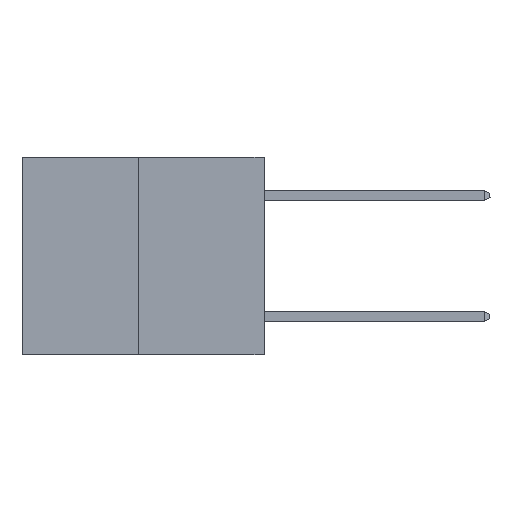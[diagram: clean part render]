
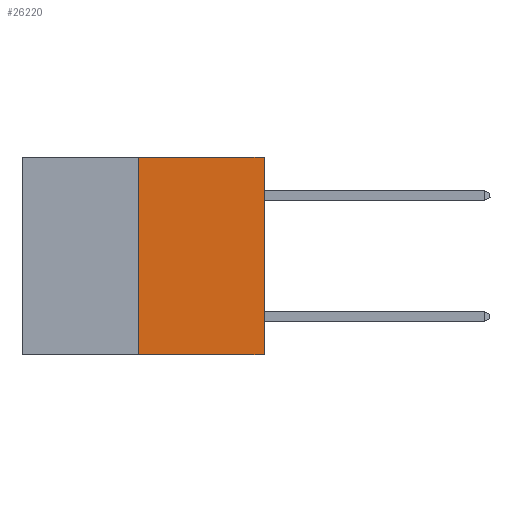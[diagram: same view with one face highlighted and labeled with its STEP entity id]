
A CAD part, left-side view. The second image highlights one B-rep face of the part: STEP entity #26220.
In plain terms, the highlighted planar face has unit normal (-1, 0, 0).
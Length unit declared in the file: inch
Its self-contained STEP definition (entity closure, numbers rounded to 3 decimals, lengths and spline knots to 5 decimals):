
#441 = LINE ( 'NONE', #14426, #9170 ) ;
#794 = DIRECTION ( 'NONE',  ( 1., 0., 0. ) ) ;
#1610 = LINE ( 'NONE', #24956, #11942 ) ;
#2062 = DIRECTION ( 'NONE',  ( 0., -1., 0. ) ) ;
#3637 = EDGE_CURVE ( 'NONE', #22764, #22365, #1610, .T. ) ;
#3825 = CARTESIAN_POINT ( 'NONE',  ( 0., 0., -0.49 ) ) ;
#4511 = ORIENTED_EDGE ( 'NONE', *, *, #6900, .F. ) ;
#5049 = ORIENTED_EDGE ( 'NONE', *, *, #18432, .T. ) ;
#6900 = EDGE_CURVE ( 'NONE', #22365, #22839, #441, .T. ) ;
#8186 = CARTESIAN_POINT ( 'NONE',  ( 0., 0., 0. ) ) ;
#9100 = VECTOR ( 'NONE', #10522, 39.37008 ) ;
#9170 = VECTOR ( 'NONE', #2062, 39.37008 ) ;
#10032 = EDGE_CURVE ( 'NONE', #21293, #22839, #24507, .T. ) ;
#10522 = DIRECTION ( 'NONE',  ( 0., -1., 0. ) ) ;
#11093 = PLANE ( 'NONE',  #14489 ) ;
#11942 = VECTOR ( 'NONE', #25140, 39.37008 ) ;
#13084 = DIRECTION ( 'NONE',  ( 0., 0., -1. ) ) ;
#14426 = CARTESIAN_POINT ( 'NONE',  ( 0., 0.6, 0. ) ) ;
#14489 = AXIS2_PLACEMENT_3D ( 'NONE', #17426, #794, #13084 ) ;
#16094 = FACE_OUTER_BOUND ( 'NONE', #24951, .T. ) ;
#17426 = CARTESIAN_POINT ( 'NONE',  ( 0., 0.6, 0. ) ) ;
#18148 = ORIENTED_EDGE ( 'NONE', *, *, #3637, .F. ) ;
#18432 = EDGE_CURVE ( 'NONE', #22764, #21293, #26215, .T. ) ;
#19176 = CARTESIAN_POINT ( 'NONE',  ( 0., 0.312, -0.49 ) ) ;
#19677 = VECTOR ( 'NONE', #24899, 39.37008 ) ;
#19795 = CARTESIAN_POINT ( 'NONE',  ( 0., 0., 0. ) ) ;
#21036 = CARTESIAN_POINT ( 'NONE',  ( 0., 0.6, -0.49 ) ) ;
#21293 = VERTEX_POINT ( 'NONE', #3825 ) ;
#22365 = VERTEX_POINT ( 'NONE', #25568 ) ;
#22570 = ORIENTED_EDGE ( 'NONE', *, *, #10032, .T. ) ;
#22764 = VERTEX_POINT ( 'NONE', #19176 ) ;
#22839 = VERTEX_POINT ( 'NONE', #19795 ) ;
#24507 = LINE ( 'NONE', #8186, #19677 ) ;
#24899 = DIRECTION ( 'NONE',  ( 0., 0., 1. ) ) ;
#24951 = EDGE_LOOP ( 'NONE', ( #18148, #5049, #22570, #4511 ) ) ;
#24956 = CARTESIAN_POINT ( 'NONE',  ( 0., 0.312, -0.49 ) ) ;
#25140 = DIRECTION ( 'NONE',  ( 0., 0., 1. ) ) ;
#25568 = CARTESIAN_POINT ( 'NONE',  ( 0., 0.312, 0. ) ) ;
#26215 = LINE ( 'NONE', #21036, #9100 ) ;
#26220 = ADVANCED_FACE ( 'NONE', ( #16094 ), #11093, .F. ) ;
